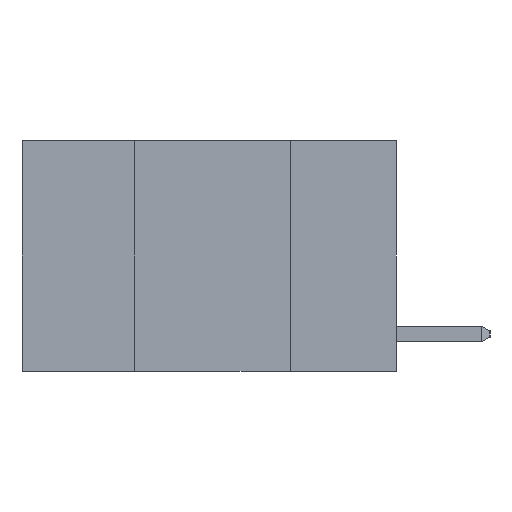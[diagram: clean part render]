
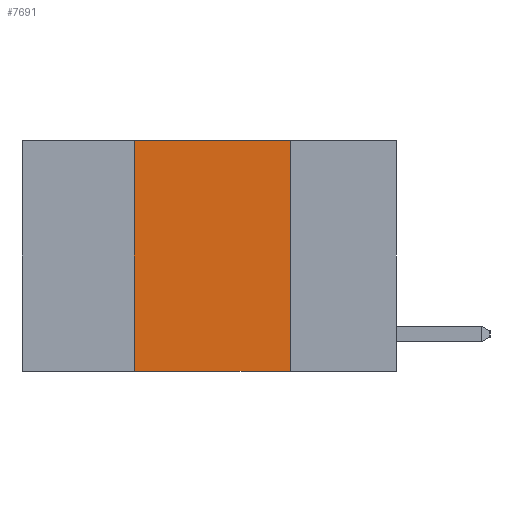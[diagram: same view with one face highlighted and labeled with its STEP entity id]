
A CAD part, left-side view. The second image highlights one B-rep face of the part: STEP entity #7691.
In plain terms, the highlighted planar face has unit normal (-1, 0, 0).
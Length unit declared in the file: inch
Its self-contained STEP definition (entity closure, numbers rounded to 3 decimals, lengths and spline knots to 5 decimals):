
#129 = EDGE_CURVE ( 'NONE', #11239, #11372, #6473, .T. ) ;
#188 = ORIENTED_EDGE ( 'NONE', *, *, #7269, .T. ) ;
#390 = EDGE_CURVE ( 'NONE', #10812, #11239, #8628, .T. ) ;
#702 = VECTOR ( 'NONE', #7065, 39.37008 ) ;
#1361 = CARTESIAN_POINT ( 'NONE',  ( 0., 0.17, 0. ) ) ;
#1710 = DIRECTION ( 'NONE',  ( 1., 0., 0. ) ) ;
#1965 = ORIENTED_EDGE ( 'NONE', *, *, #3252, .F. ) ;
#2357 = VERTEX_POINT ( 'NONE', #5288 ) ;
#2817 = LINE ( 'NONE', #10882, #10663 ) ;
#3252 = EDGE_CURVE ( 'NONE', #2357, #10812, #11170, .T. ) ;
#3680 = CARTESIAN_POINT ( 'NONE',  ( 0., 0.6, 0. ) ) ;
#3750 = CARTESIAN_POINT ( 'NONE',  ( 0., 0.42, 0. ) ) ;
#4675 = PLANE ( 'NONE',  #11908 ) ;
#5182 = ORIENTED_EDGE ( 'NONE', *, *, #129, .F. ) ;
#5288 = CARTESIAN_POINT ( 'NONE',  ( 0., 0.42, -0.37 ) ) ;
#5744 = FACE_OUTER_BOUND ( 'NONE', #10646, .T. ) ;
#5798 = CARTESIAN_POINT ( 'NONE',  ( 0., 0.17, 0. ) ) ;
#6473 = LINE ( 'NONE', #5798, #8793 ) ;
#7065 = DIRECTION ( 'NONE',  ( 0., -1., 0. ) ) ;
#7269 = EDGE_CURVE ( 'NONE', #2357, #11372, #2817, .T. ) ;
#7670 = CARTESIAN_POINT ( 'NONE',  ( 0., 0.17, -0.37 ) ) ;
#7691 = ADVANCED_FACE ( 'NONE', ( #5744 ), #4675, .F. ) ;
#7919 = DIRECTION ( 'NONE',  ( 0., -1., 0. ) ) ;
#8563 = VECTOR ( 'NONE', #9571, 39.37008 ) ;
#8607 = DIRECTION ( 'NONE',  ( 0., 0., -1. ) ) ;
#8628 = LINE ( 'NONE', #11019, #702 ) ;
#8793 = VECTOR ( 'NONE', #9082, 39.37008 ) ;
#9082 = DIRECTION ( 'NONE',  ( 0., 0., -1. ) ) ;
#9571 = DIRECTION ( 'NONE',  ( 0., 0., 1. ) ) ;
#10259 = ORIENTED_EDGE ( 'NONE', *, *, #390, .F. ) ;
#10527 = CARTESIAN_POINT ( 'NONE',  ( 0., 0.42, 0. ) ) ;
#10646 = EDGE_LOOP ( 'NONE', ( #5182, #10259, #1965, #188 ) ) ;
#10663 = VECTOR ( 'NONE', #7919, 39.37008 ) ;
#10812 = VERTEX_POINT ( 'NONE', #3750 ) ;
#10882 = CARTESIAN_POINT ( 'NONE',  ( 0., 0.6, -0.37 ) ) ;
#11019 = CARTESIAN_POINT ( 'NONE',  ( 0., 0.6, 0. ) ) ;
#11170 = LINE ( 'NONE', #10527, #8563 ) ;
#11239 = VERTEX_POINT ( 'NONE', #1361 ) ;
#11372 = VERTEX_POINT ( 'NONE', #7670 ) ;
#11908 = AXIS2_PLACEMENT_3D ( 'NONE', #3680, #1710, #8607 ) ;
